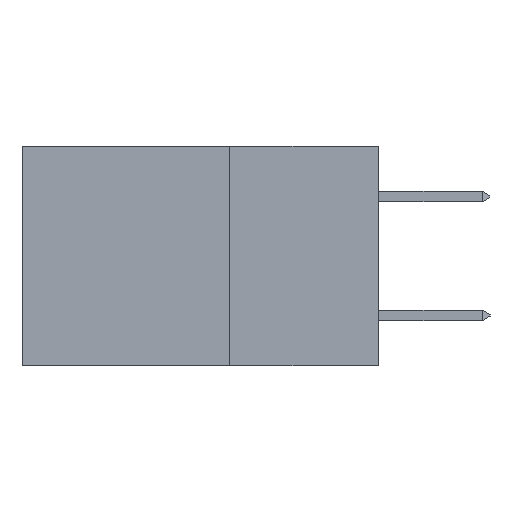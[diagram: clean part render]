
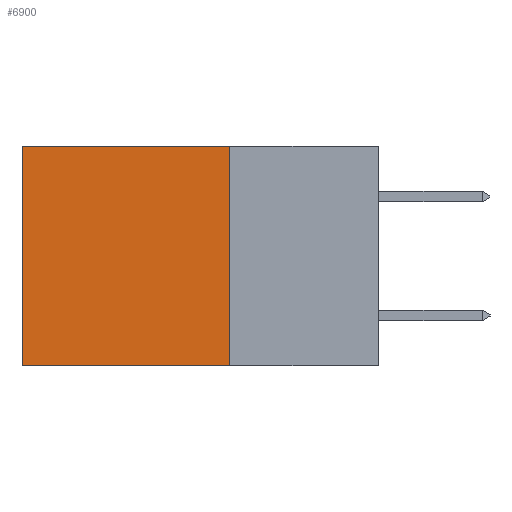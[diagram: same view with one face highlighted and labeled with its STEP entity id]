
A CAD part, left-side view. The second image highlights one B-rep face of the part: STEP entity #6900.
In plain terms, the highlighted planar face has unit normal (-1, 0, 0).
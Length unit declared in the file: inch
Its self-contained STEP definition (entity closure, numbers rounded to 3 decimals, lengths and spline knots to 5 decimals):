
#93 = VECTOR ( 'NONE', #1821, 39.37008 ) ;
#976 = VERTEX_POINT ( 'NONE', #13312 ) ;
#1147 = CARTESIAN_POINT ( 'NONE',  ( 0.2615, 0.25, 0. ) ) ;
#1656 = FACE_OUTER_BOUND ( 'NONE', #11678, .T. ) ;
#1821 = DIRECTION ( 'NONE',  ( 0., 1., 0. ) ) ;
#2249 = EDGE_CURVE ( 'NONE', #13555, #5696, #13154, .T. ) ;
#2708 = VECTOR ( 'NONE', #9263, 39.37008 ) ;
#2915 = CARTESIAN_POINT ( 'NONE',  ( 0.2615, 0.25, 0. ) ) ;
#2948 = DIRECTION ( 'NONE',  ( 0., 0., -1. ) ) ;
#3000 = DIRECTION ( 'NONE',  ( 1., 0., 0. ) ) ;
#3099 = DIRECTION ( 'NONE',  ( 0., 0., -1. ) ) ;
#3113 = EDGE_CURVE ( 'NONE', #976, #5360, #14806, .T. ) ;
#3235 = LINE ( 'NONE', #1147, #93 ) ;
#3318 = CARTESIAN_POINT ( 'NONE',  ( 0.2615, 0.25, -0.37 ) ) ;
#3329 = PLANE ( 'NONE',  #4770 ) ;
#3544 = LINE ( 'NONE', #6569, #12369 ) ;
#3765 = EDGE_CURVE ( 'NONE', #13555, #976, #3235, .T. ) ;
#4770 = AXIS2_PLACEMENT_3D ( 'NONE', #3318, #3000, #2948 ) ;
#5360 = VERTEX_POINT ( 'NONE', #6011 ) ;
#5544 = ORIENTED_EDGE ( 'NONE', *, *, #2249, .F. ) ;
#5696 = VERTEX_POINT ( 'NONE', #13542 ) ;
#6011 = CARTESIAN_POINT ( 'NONE',  ( 0.2615, 0.6, -0.37 ) ) ;
#6487 = DIRECTION ( 'NONE',  ( 0., 1., 0. ) ) ;
#6569 = CARTESIAN_POINT ( 'NONE',  ( 0.2615, 0.25, -0.37 ) ) ;
#6900 = ADVANCED_FACE ( 'NONE', ( #1656 ), #3329, .F. ) ;
#7438 = VECTOR ( 'NONE', #3099, 39.37008 ) ;
#7734 = CARTESIAN_POINT ( 'NONE',  ( 0.2615, 0.25, -0.37 ) ) ;
#8855 = CARTESIAN_POINT ( 'NONE',  ( 0.2615, 0.6, -0.37 ) ) ;
#9263 = DIRECTION ( 'NONE',  ( 0., 0., -1. ) ) ;
#10804 = ORIENTED_EDGE ( 'NONE', *, *, #3113, .T. ) ;
#11678 = EDGE_LOOP ( 'NONE', ( #10804, #13010, #5544, #13671 ) ) ;
#12369 = VECTOR ( 'NONE', #6487, 39.37008 ) ;
#12975 = EDGE_CURVE ( 'NONE', #5696, #5360, #3544, .T. ) ;
#13010 = ORIENTED_EDGE ( 'NONE', *, *, #12975, .F. ) ;
#13154 = LINE ( 'NONE', #7734, #7438 ) ;
#13312 = CARTESIAN_POINT ( 'NONE',  ( 0.2615, 0.6, 0. ) ) ;
#13542 = CARTESIAN_POINT ( 'NONE',  ( 0.2615, 0.25, -0.37 ) ) ;
#13555 = VERTEX_POINT ( 'NONE', #2915 ) ;
#13671 = ORIENTED_EDGE ( 'NONE', *, *, #3765, .T. ) ;
#14806 = LINE ( 'NONE', #8855, #2708 ) ;
